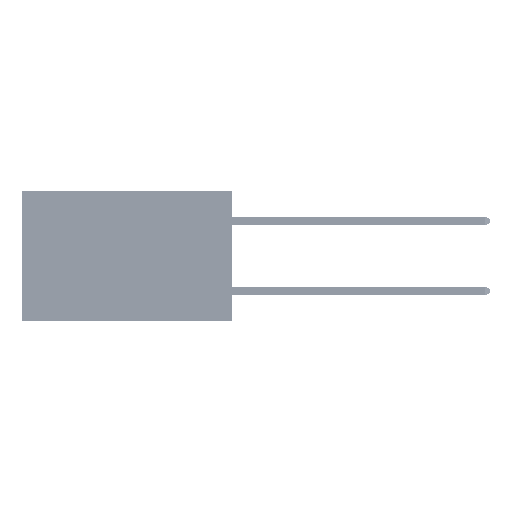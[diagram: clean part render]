
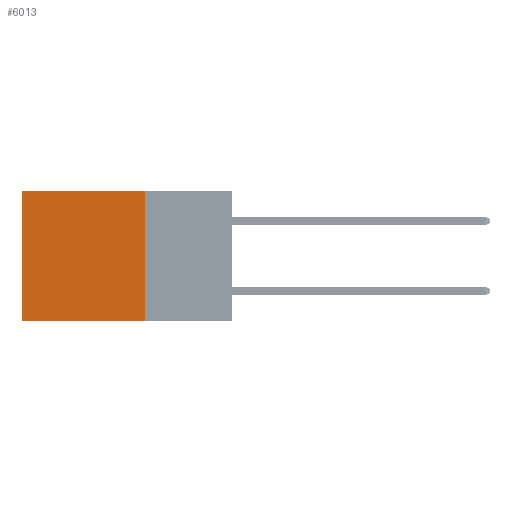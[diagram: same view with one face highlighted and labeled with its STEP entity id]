
A CAD part, left-side view. The second image highlights one B-rep face of the part: STEP entity #6013.
In plain terms, the highlighted planar face has unit normal (-1, 0, 0).
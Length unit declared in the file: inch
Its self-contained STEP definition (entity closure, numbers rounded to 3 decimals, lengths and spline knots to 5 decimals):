
#1815 = VERTEX_POINT ( 'NONE', #17097 ) ;
#2554 = EDGE_CURVE ( 'NONE', #4936, #3045, #36656, .T. ) ;
#3045 = VERTEX_POINT ( 'NONE', #28275 ) ;
#3716 = LINE ( 'NONE', #27378, #13362 ) ;
#4521 = ORIENTED_EDGE ( 'NONE', *, *, #33084, .F. ) ;
#4670 = EDGE_CURVE ( 'NONE', #1815, #36174, #15946, .T. ) ;
#4936 = VERTEX_POINT ( 'NONE', #27038 ) ;
#5449 = DIRECTION ( 'NONE',  ( 0., 0., -1. ) ) ;
#6013 = ADVANCED_FACE ( 'NONE', ( #17806 ), #17669, .F. ) ;
#7113 = DIRECTION ( 'NONE',  ( 0., 0., -1. ) ) ;
#13226 = CARTESIAN_POINT ( 'NONE',  ( 0.2875, 0.25, 0. ) ) ;
#13362 = VECTOR ( 'NONE', #39732, 39.37008 ) ;
#15206 = CARTESIAN_POINT ( 'NONE',  ( 0.2875, 0.6, 0. ) ) ;
#15946 = LINE ( 'NONE', #25443, #47242 ) ;
#16036 = EDGE_CURVE ( 'NONE', #3045, #36174, #24267, .T. ) ;
#17097 = CARTESIAN_POINT ( 'NONE',  ( 0.2875, 0.25, -0.37 ) ) ;
#17407 = ORIENTED_EDGE ( 'NONE', *, *, #4670, .F. ) ;
#17669 = PLANE ( 'NONE',  #52257 ) ;
#17806 = FACE_OUTER_BOUND ( 'NONE', #19527, .T. ) ;
#19527 = EDGE_LOOP ( 'NONE', ( #41601, #17407, #4521, #47239 ) ) ;
#21336 = DIRECTION ( 'NONE',  ( 0., 1., 0. ) ) ;
#21469 = DIRECTION ( 'NONE',  ( 0., 1., 0. ) ) ;
#24267 = LINE ( 'NONE', #15206, #42180 ) ;
#25443 = CARTESIAN_POINT ( 'NONE',  ( 0.2875, 0.25, -0.37 ) ) ;
#25769 = VECTOR ( 'NONE', #21469, 39.37008 ) ;
#25869 = CARTESIAN_POINT ( 'NONE',  ( 0.2875, 0.25, 0. ) ) ;
#27038 = CARTESIAN_POINT ( 'NONE',  ( 0.2875, 0.25, 0. ) ) ;
#27378 = CARTESIAN_POINT ( 'NONE',  ( 0.2875, 0.25, 0. ) ) ;
#28275 = CARTESIAN_POINT ( 'NONE',  ( 0.2875, 0.6, 0. ) ) ;
#29969 = DIRECTION ( 'NONE',  ( 1., 0., 0. ) ) ;
#33084 = EDGE_CURVE ( 'NONE', #4936, #1815, #3716, .T. ) ;
#36174 = VERTEX_POINT ( 'NONE', #37511 ) ;
#36656 = LINE ( 'NONE', #13226, #25769 ) ;
#37511 = CARTESIAN_POINT ( 'NONE',  ( 0.2875, 0.6, -0.37 ) ) ;
#39732 = DIRECTION ( 'NONE',  ( 0., 0., -1. ) ) ;
#41601 = ORIENTED_EDGE ( 'NONE', *, *, #16036, .T. ) ;
#42180 = VECTOR ( 'NONE', #7113, 39.37008 ) ;
#47239 = ORIENTED_EDGE ( 'NONE', *, *, #2554, .T. ) ;
#47242 = VECTOR ( 'NONE', #21336, 39.37008 ) ;
#52257 = AXIS2_PLACEMENT_3D ( 'NONE', #25869, #29969, #5449 ) ;
